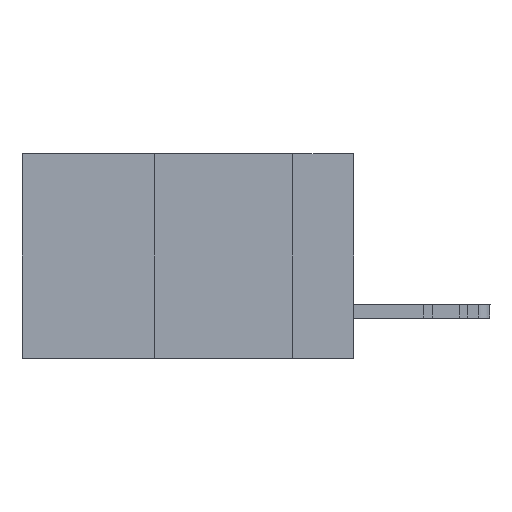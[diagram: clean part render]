
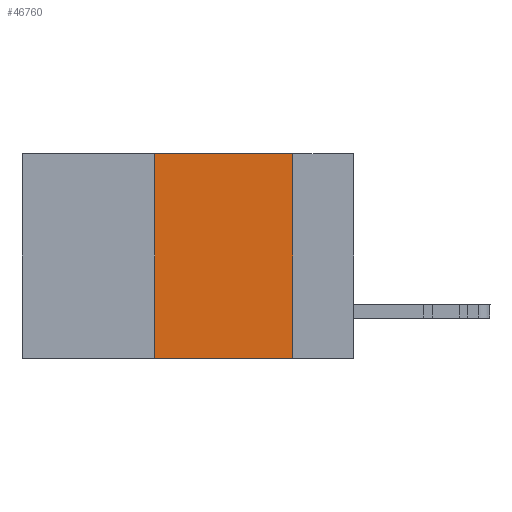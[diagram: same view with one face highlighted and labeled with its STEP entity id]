
A CAD part, left-side view. The second image highlights one B-rep face of the part: STEP entity #46760.
In plain terms, the highlighted planar face has unit normal (-1, 0, 0).
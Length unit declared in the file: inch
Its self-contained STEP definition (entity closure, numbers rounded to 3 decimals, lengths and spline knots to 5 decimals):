
#497 = CARTESIAN_POINT ( 'NONE',  ( 0., 0.6, 0. ) ) ;
#2475 = EDGE_CURVE ( 'NONE', #46253, #6562, #45811, .T. ) ;
#4066 = EDGE_CURVE ( 'NONE', #46253, #27688, #16666, .T. ) ;
#5154 = DIRECTION ( 'NONE',  ( 0., 0., 1. ) ) ;
#5508 = LINE ( 'NONE', #42409, #30102 ) ;
#6562 = VERTEX_POINT ( 'NONE', #45727 ) ;
#8020 = VECTOR ( 'NONE', #29882, 39.37008 ) ;
#8663 = AXIS2_PLACEMENT_3D ( 'NONE', #29671, #33775, #15454 ) ;
#11364 = ORIENTED_EDGE ( 'NONE', *, *, #27776, .F. ) ;
#12020 = DIRECTION ( 'NONE',  ( 0., -1., 0. ) ) ;
#12091 = EDGE_LOOP ( 'NONE', ( #13224, #11364, #13043, #44821 ) ) ;
#13043 = ORIENTED_EDGE ( 'NONE', *, *, #4066, .F. ) ;
#13224 = ORIENTED_EDGE ( 'NONE', *, *, #14766, .F. ) ;
#14766 = EDGE_CURVE ( 'NONE', #28922, #6562, #5508, .T. ) ;
#15131 = VECTOR ( 'NONE', #5154, 39.37008 ) ;
#15192 = CARTESIAN_POINT ( 'NONE',  ( 0., 0.36, 0. ) ) ;
#15454 = DIRECTION ( 'NONE',  ( 0., 0., -1. ) ) ;
#16056 = DIRECTION ( 'NONE',  ( 0., 0., -1. ) ) ;
#16666 = LINE ( 'NONE', #38147, #15131 ) ;
#18219 = CARTESIAN_POINT ( 'NONE',  ( 0., 0.36, -0.37 ) ) ;
#21902 = VECTOR ( 'NONE', #12020, 39.37008 ) ;
#23381 = FACE_OUTER_BOUND ( 'NONE', #12091, .T. ) ;
#27688 = VERTEX_POINT ( 'NONE', #15192 ) ;
#27776 = EDGE_CURVE ( 'NONE', #27688, #28922, #37618, .T. ) ;
#28922 = VERTEX_POINT ( 'NONE', #40094 ) ;
#29671 = CARTESIAN_POINT ( 'NONE',  ( 0., 0.6, 0. ) ) ;
#29882 = DIRECTION ( 'NONE',  ( 0., -1., 0. ) ) ;
#30102 = VECTOR ( 'NONE', #16056, 39.37008 ) ;
#33308 = PLANE ( 'NONE',  #8663 ) ;
#33775 = DIRECTION ( 'NONE',  ( 1., 0., 0. ) ) ;
#37618 = LINE ( 'NONE', #497, #8020 ) ;
#38147 = CARTESIAN_POINT ( 'NONE',  ( 0., 0.36, 0. ) ) ;
#40094 = CARTESIAN_POINT ( 'NONE',  ( 0., 0.11, 0. ) ) ;
#42409 = CARTESIAN_POINT ( 'NONE',  ( 0., 0.11, 0. ) ) ;
#44821 = ORIENTED_EDGE ( 'NONE', *, *, #2475, .T. ) ;
#45086 = CARTESIAN_POINT ( 'NONE',  ( 0., 0.6, -0.37 ) ) ;
#45727 = CARTESIAN_POINT ( 'NONE',  ( 0., 0.11, -0.37 ) ) ;
#45811 = LINE ( 'NONE', #45086, #21902 ) ;
#46253 = VERTEX_POINT ( 'NONE', #18219 ) ;
#46760 = ADVANCED_FACE ( 'NONE', ( #23381 ), #33308, .F. ) ;
